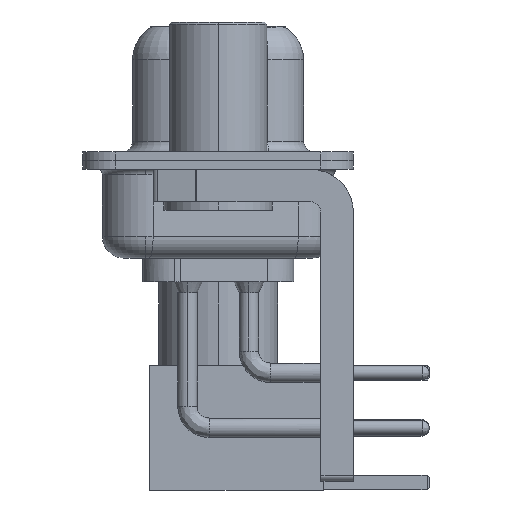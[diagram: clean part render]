
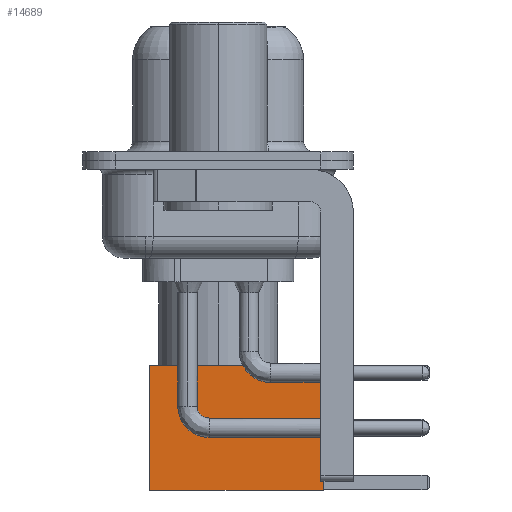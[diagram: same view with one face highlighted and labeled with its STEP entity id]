
A CAD part, left-side view. The second image highlights one B-rep face of the part: STEP entity #14689.
In plain terms, the highlighted face is planar.
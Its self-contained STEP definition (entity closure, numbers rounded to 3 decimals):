
#520 = VECTOR ( 'NONE', #22028, 1000. ) ;
#996 = CARTESIAN_POINT ( 'NONE',  ( 2.875, 2.875, 8. ) ) ;
#2361 = DIRECTION ( 'NONE',  ( -1., 0., 0. ) ) ;
#2951 = VECTOR ( 'NONE', #13321, 1000. ) ;
#3184 = CARTESIAN_POINT ( 'NONE',  ( 0., 2.875, 0. ) ) ;
#3185 = VECTOR ( 'NONE', #2361, 1000. ) ;
#4669 = CARTESIAN_POINT ( 'NONE',  ( -2.875, 2.875, 8. ) ) ;
#5808 = CARTESIAN_POINT ( 'NONE',  ( 2.875, 2.875, 0. ) ) ;
#6018 = LINE ( 'NONE', #7732, #3185 ) ;
#6158 = VERTEX_POINT ( 'NONE', #23635 ) ;
#6321 = EDGE_CURVE ( 'NONE', #6158, #6955, #7094, .T. ) ;
#6955 = VERTEX_POINT ( 'NONE', #17488 ) ;
#7094 = LINE ( 'NONE', #3184, #520 ) ;
#7732 = CARTESIAN_POINT ( 'NONE',  ( 0., 2.875, 8. ) ) ;
#8382 = ORIENTED_EDGE ( 'NONE', *, *, #13076, .F. ) ;
#8931 = CARTESIAN_POINT ( 'NONE',  ( 2.875, 2.875, 0. ) ) ;
#9856 = LINE ( 'NONE', #5808, #2951 ) ;
#10279 = CARTESIAN_POINT ( 'NONE',  ( -2.875, 2.875, 0. ) ) ;
#11029 = PLANE ( 'NONE',  #19358 ) ;
#11973 = VERTEX_POINT ( 'NONE', #996 ) ;
#13076 = EDGE_CURVE ( 'NONE', #11973, #14645, #6018, .T. ) ;
#13234 = EDGE_LOOP ( 'NONE', ( #18118, #19802, #19214, #8382 ) ) ;
#13321 = DIRECTION ( 'NONE',  ( 0., 0., -1. ) ) ;
#13862 = VECTOR ( 'NONE', #17950, 1000. ) ;
#14645 = VERTEX_POINT ( 'NONE', #4669 ) ;
#14689 = ADVANCED_FACE ( 'NONE', ( #18343 ), #11029, .T. ) ;
#14989 = EDGE_CURVE ( 'NONE', #14645, #6955, #17579, .T. ) ;
#17300 = EDGE_CURVE ( 'NONE', #11973, #6158, #9856, .T. ) ;
#17488 = CARTESIAN_POINT ( 'NONE',  ( -2.875, 2.875, 0. ) ) ;
#17579 = LINE ( 'NONE', #10279, #13862 ) ;
#17950 = DIRECTION ( 'NONE',  ( 0., 0., -1. ) ) ;
#18118 = ORIENTED_EDGE ( 'NONE', *, *, #17300, .T. ) ;
#18343 = FACE_OUTER_BOUND ( 'NONE', #13234, .T. ) ;
#19214 = ORIENTED_EDGE ( 'NONE', *, *, #14989, .F. ) ;
#19358 = AXIS2_PLACEMENT_3D ( 'NONE', #8931, #20665, #20190 ) ;
#19802 = ORIENTED_EDGE ( 'NONE', *, *, #6321, .T. ) ;
#20190 = DIRECTION ( 'NONE',  ( 0., 0., 1. ) ) ;
#20665 = DIRECTION ( 'NONE',  ( 0., 1., 0. ) ) ;
#22028 = DIRECTION ( 'NONE',  ( -1., 0., 0. ) ) ;
#23635 = CARTESIAN_POINT ( 'NONE',  ( 2.875, 2.875, 0. ) ) ;
